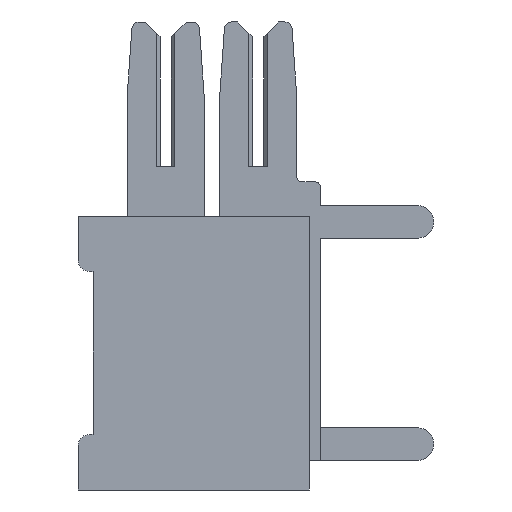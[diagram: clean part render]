
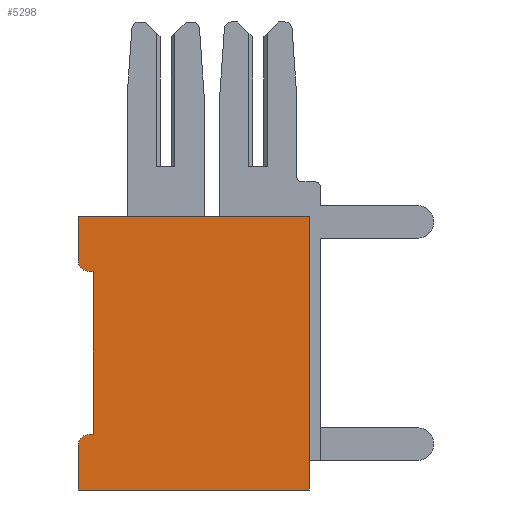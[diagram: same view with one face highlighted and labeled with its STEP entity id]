
A CAD part, left-side view. The second image highlights one B-rep face of the part: STEP entity #5298.
In plain terms, the highlighted planar face has unit normal (-1, 0, 0).
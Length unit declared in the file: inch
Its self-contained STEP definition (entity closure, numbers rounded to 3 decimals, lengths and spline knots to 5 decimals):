
#147 = CARTESIAN_POINT ( 'NONE',  ( 0., 0.292, -0.075 ) ) ;
#414 = VECTOR ( 'NONE', #10465, 39.37008 ) ;
#551 = CARTESIAN_POINT ( 'NONE',  ( 0., 0., -0.37 ) ) ;
#675 = VECTOR ( 'NONE', #1924, 39.37008 ) ;
#877 = CARTESIAN_POINT ( 'NONE',  ( 0., 0., -0.37 ) ) ;
#1188 = VECTOR ( 'NONE', #5732, 39.37008 ) ;
#1379 = CARTESIAN_POINT ( 'NONE',  ( 0., 0.312, -0.37 ) ) ;
#1397 = ORIENTED_EDGE ( 'NONE', *, *, #1494, .F. ) ;
#1476 = VECTOR ( 'NONE', #2235, 39.37008 ) ;
#1494 = EDGE_CURVE ( 'NONE', #7544, #6524, #4221, .T. ) ;
#1552 = DIRECTION ( 'NONE',  ( -1., 0., 0. ) ) ;
#1892 = CIRCLE ( 'NONE', #2628, 0.015 ) ;
#1924 = DIRECTION ( 'NONE',  ( 0., 1., 0. ) ) ;
#2038 = CARTESIAN_POINT ( 'NONE',  ( 0., 0.312, -0.075 ) ) ;
#2149 = DIRECTION ( 'NONE',  ( 0., 0., 1. ) ) ;
#2235 = DIRECTION ( 'NONE',  ( 0., -1., 0. ) ) ;
#2250 = CIRCLE ( 'NONE', #5963, 0.015 ) ;
#2309 = EDGE_CURVE ( 'NONE', #8614, #5224, #2250, .T. ) ;
#2502 = EDGE_CURVE ( 'NONE', #6965, #8590, #9306, .T. ) ;
#2525 = DIRECTION ( 'NONE',  ( 0., 0., 1. ) ) ;
#2597 = PLANE ( 'NONE',  #9906 ) ;
#2628 = AXIS2_PLACEMENT_3D ( 'NONE', #4205, #1552, #7391 ) ;
#2694 = EDGE_CURVE ( 'NONE', #5075, #7544, #4864, .T. ) ;
#2808 = EDGE_CURVE ( 'NONE', #10723, #9366, #10081, .T. ) ;
#2873 = CARTESIAN_POINT ( 'NONE',  ( 0., 0.312, -0.37 ) ) ;
#2889 = DIRECTION ( 'NONE',  ( 0., -1., 0. ) ) ;
#2943 = LINE ( 'NONE', #6750, #5938 ) ;
#3344 = CARTESIAN_POINT ( 'NONE',  ( 0., 0., 0. ) ) ;
#3583 = CARTESIAN_POINT ( 'NONE',  ( 0., 0.312, 0. ) ) ;
#3786 = ORIENTED_EDGE ( 'NONE', *, *, #2502, .T. ) ;
#3986 = ORIENTED_EDGE ( 'NONE', *, *, #10773, .T. ) ;
#4034 = ORIENTED_EDGE ( 'NONE', *, *, #2309, .T. ) ;
#4205 = CARTESIAN_POINT ( 'NONE',  ( 0., 0.297, -0.06 ) ) ;
#4221 = LINE ( 'NONE', #7773, #9462 ) ;
#4304 = VERTEX_POINT ( 'NONE', #8189 ) ;
#4314 = CARTESIAN_POINT ( 'NONE',  ( 0., 0.312, -0.31 ) ) ;
#4446 = EDGE_LOOP ( 'NONE', ( #10831, #8600, #9153, #10184, #6468, #4034, #8698, #3786, #3986, #1397 ) ) ;
#4851 = CARTESIAN_POINT ( 'NONE',  ( 0., 0., -0.37 ) ) ;
#4864 = LINE ( 'NONE', #8925, #414 ) ;
#4895 = CARTESIAN_POINT ( 'NONE',  ( 0., 0.292, -0.295 ) ) ;
#4980 = CARTESIAN_POINT ( 'NONE',  ( 0., 0.297, -0.295 ) ) ;
#5049 = CARTESIAN_POINT ( 'NONE',  ( 0., 0., -0.37 ) ) ;
#5075 = VERTEX_POINT ( 'NONE', #6619 ) ;
#5224 = VERTEX_POINT ( 'NONE', #4314 ) ;
#5298 = ADVANCED_FACE ( 'NONE', ( #7710 ), #2597, .T. ) ;
#5732 = DIRECTION ( 'NONE',  ( 0., 0., 1. ) ) ;
#5938 = VECTOR ( 'NONE', #8416, 39.37008 ) ;
#5963 = AXIS2_PLACEMENT_3D ( 'NONE', #8857, #6290, #9773 ) ;
#6290 = DIRECTION ( 'NONE',  ( -1., 0., 0. ) ) ;
#6377 = CARTESIAN_POINT ( 'NONE',  ( 0., 0.292, -0.295 ) ) ;
#6468 = ORIENTED_EDGE ( 'NONE', *, *, #7145, .F. ) ;
#6524 = VERTEX_POINT ( 'NONE', #3344 ) ;
#6619 = CARTESIAN_POINT ( 'NONE',  ( 0., 0.312, -0.06 ) ) ;
#6750 = CARTESIAN_POINT ( 'NONE',  ( 0., 0.312, -0.295 ) ) ;
#6965 = VERTEX_POINT ( 'NONE', #2873 ) ;
#7118 = LINE ( 'NONE', #1379, #9747 ) ;
#7126 = EDGE_CURVE ( 'NONE', #5075, #4304, #1892, .T. ) ;
#7145 = EDGE_CURVE ( 'NONE', #8614, #10723, #2943, .T. ) ;
#7387 = EDGE_CURVE ( 'NONE', #6965, #5224, #7118, .T. ) ;
#7391 = DIRECTION ( 'NONE',  ( 0., 0., 1. ) ) ;
#7544 = VERTEX_POINT ( 'NONE', #3583 ) ;
#7710 = FACE_OUTER_BOUND ( 'NONE', #4446, .T. ) ;
#7773 = CARTESIAN_POINT ( 'NONE',  ( 0., 0., 0. ) ) ;
#8189 = CARTESIAN_POINT ( 'NONE',  ( 0., 0.297, -0.075 ) ) ;
#8416 = DIRECTION ( 'NONE',  ( 0., -1., 0. ) ) ;
#8590 = VERTEX_POINT ( 'NONE', #5049 ) ;
#8600 = ORIENTED_EDGE ( 'NONE', *, *, #7126, .T. ) ;
#8614 = VERTEX_POINT ( 'NONE', #4980 ) ;
#8698 = ORIENTED_EDGE ( 'NONE', *, *, #7387, .F. ) ;
#8857 = CARTESIAN_POINT ( 'NONE',  ( 0., 0.297, -0.31 ) ) ;
#8925 = CARTESIAN_POINT ( 'NONE',  ( 0., 0.312, -0.37 ) ) ;
#9046 = LINE ( 'NONE', #2038, #675 ) ;
#9153 = ORIENTED_EDGE ( 'NONE', *, *, #10275, .F. ) ;
#9293 = LINE ( 'NONE', #4851, #10751 ) ;
#9306 = LINE ( 'NONE', #551, #1476 ) ;
#9366 = VERTEX_POINT ( 'NONE', #147 ) ;
#9462 = VECTOR ( 'NONE', #2889, 39.37008 ) ;
#9747 = VECTOR ( 'NONE', #2149, 39.37008 ) ;
#9755 = DIRECTION ( 'NONE',  ( 0., 0., 1. ) ) ;
#9773 = DIRECTION ( 'NONE',  ( 0., 0., 1. ) ) ;
#9906 = AXIS2_PLACEMENT_3D ( 'NONE', #877, #10123, #2525 ) ;
#10081 = LINE ( 'NONE', #4895, #1188 ) ;
#10123 = DIRECTION ( 'NONE',  ( -1., 0., 0. ) ) ;
#10184 = ORIENTED_EDGE ( 'NONE', *, *, #2808, .F. ) ;
#10275 = EDGE_CURVE ( 'NONE', #9366, #4304, #9046, .T. ) ;
#10465 = DIRECTION ( 'NONE',  ( 0., 0., 1. ) ) ;
#10723 = VERTEX_POINT ( 'NONE', #6377 ) ;
#10751 = VECTOR ( 'NONE', #9755, 39.37008 ) ;
#10773 = EDGE_CURVE ( 'NONE', #8590, #6524, #9293, .T. ) ;
#10831 = ORIENTED_EDGE ( 'NONE', *, *, #2694, .F. ) ;
